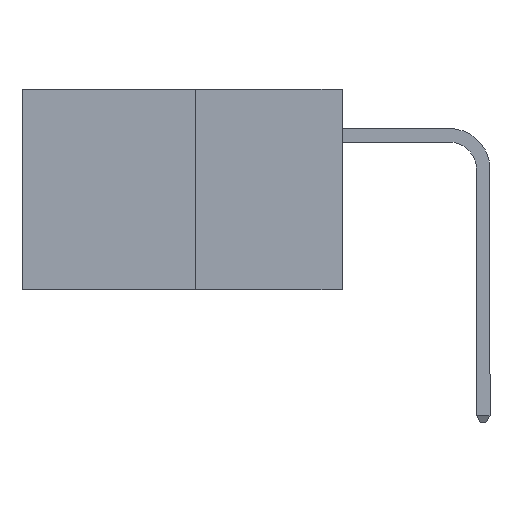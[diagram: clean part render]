
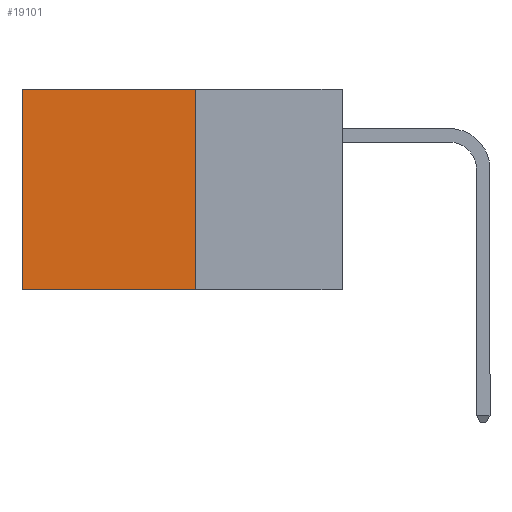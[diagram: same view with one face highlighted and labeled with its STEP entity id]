
A CAD part, left-side view. The second image highlights one B-rep face of the part: STEP entity #19101.
In plain terms, the highlighted planar face has unit normal (-1, 0, 0).
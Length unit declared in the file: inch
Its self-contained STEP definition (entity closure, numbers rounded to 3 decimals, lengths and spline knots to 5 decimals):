
#477 = CARTESIAN_POINT ( 'NONE',  ( 0.277, 0.27, -0.37 ) ) ;
#1582 = CARTESIAN_POINT ( 'NONE',  ( 0.277, 0.27, 0. ) ) ;
#1772 = VECTOR ( 'NONE', #12776, 39.37008 ) ;
#2138 = VECTOR ( 'NONE', #16195, 39.37008 ) ;
#4156 = DIRECTION ( 'NONE',  ( 0., 0., -1. ) ) ;
#5155 = FACE_OUTER_BOUND ( 'NONE', #18872, .T. ) ;
#5377 = CARTESIAN_POINT ( 'NONE',  ( 0.277, 0.27, -0.37 ) ) ;
#6293 = CARTESIAN_POINT ( 'NONE',  ( 0.277, 0.59, -0.37 ) ) ;
#6575 = ORIENTED_EDGE ( 'NONE', *, *, #10616, .F. ) ;
#7187 = VERTEX_POINT ( 'NONE', #6293 ) ;
#7571 = EDGE_CURVE ( 'NONE', #15008, #16821, #16378, .T. ) ;
#8713 = ORIENTED_EDGE ( 'NONE', *, *, #10817, .F. ) ;
#9441 = DIRECTION ( 'NONE',  ( 0., 0., -1. ) ) ;
#10616 = EDGE_CURVE ( 'NONE', #15008, #18947, #10628, .T. ) ;
#10628 = LINE ( 'NONE', #21880, #19470 ) ;
#10817 = EDGE_CURVE ( 'NONE', #18947, #7187, #19187, .T. ) ;
#11005 = CARTESIAN_POINT ( 'NONE',  ( 0.277, 0.59, -0.37 ) ) ;
#12026 = DIRECTION ( 'NONE',  ( 0., 1., 0. ) ) ;
#12665 = CARTESIAN_POINT ( 'NONE',  ( 0.277, 0.27, 0. ) ) ;
#12776 = DIRECTION ( 'NONE',  ( 0., 0., -1. ) ) ;
#13317 = EDGE_CURVE ( 'NONE', #16821, #7187, #16015, .T. ) ;
#13330 = CARTESIAN_POINT ( 'NONE',  ( 0.277, 0.59, 0. ) ) ;
#15008 = VERTEX_POINT ( 'NONE', #1582 ) ;
#15035 = VECTOR ( 'NONE', #12026, 39.37008 ) ;
#16015 = LINE ( 'NONE', #11005, #1772 ) ;
#16195 = DIRECTION ( 'NONE',  ( 0., 1., 0. ) ) ;
#16378 = LINE ( 'NONE', #12665, #2138 ) ;
#16821 = VERTEX_POINT ( 'NONE', #13330 ) ;
#16924 = ORIENTED_EDGE ( 'NONE', *, *, #7571, .T. ) ;
#18318 = PLANE ( 'NONE',  #22241 ) ;
#18872 = EDGE_LOOP ( 'NONE', ( #20429, #8713, #6575, #16924 ) ) ;
#18947 = VERTEX_POINT ( 'NONE', #5377 ) ;
#19101 = ADVANCED_FACE ( 'NONE', ( #5155 ), #18318, .F. ) ;
#19187 = LINE ( 'NONE', #22540, #15035 ) ;
#19470 = VECTOR ( 'NONE', #4156, 39.37008 ) ;
#20099 = DIRECTION ( 'NONE',  ( 1., 0., 0. ) ) ;
#20429 = ORIENTED_EDGE ( 'NONE', *, *, #13317, .T. ) ;
#21880 = CARTESIAN_POINT ( 'NONE',  ( 0.277, 0.27, -0.37 ) ) ;
#22241 = AXIS2_PLACEMENT_3D ( 'NONE', #477, #20099, #9441 ) ;
#22540 = CARTESIAN_POINT ( 'NONE',  ( 0.277, 0.27, -0.37 ) ) ;
